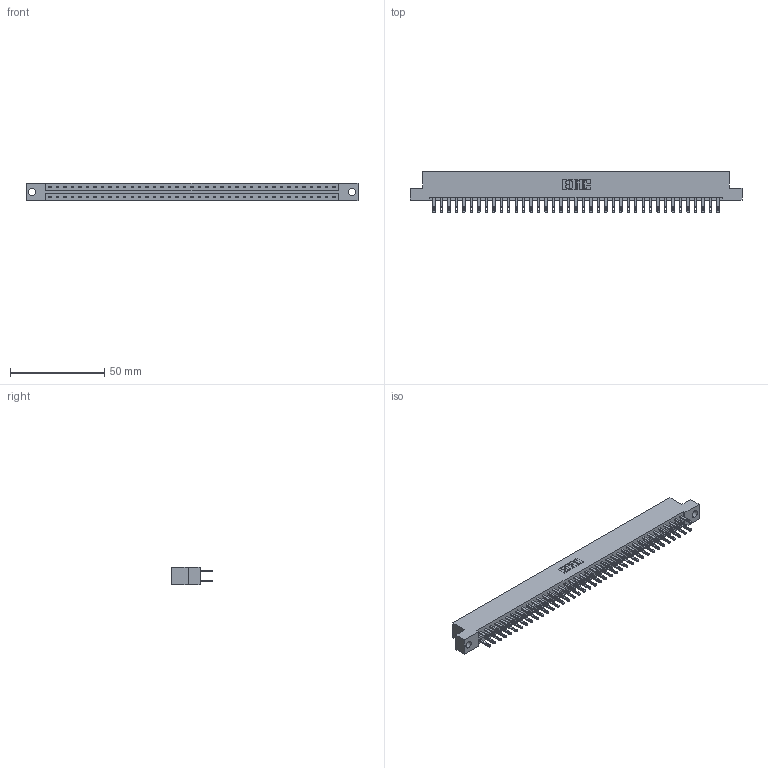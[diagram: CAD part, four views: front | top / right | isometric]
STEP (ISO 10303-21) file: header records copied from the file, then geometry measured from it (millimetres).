
FILE_DESCRIPTION (( 'STEP AP203' ), '1' );
FILE_NAME ('333-078-500-204.STEP', '2018-08-04T23:46:27', ( '' ), ( '' ), 'SwSTEP 2.0', 'SolidWorks 2016', '' );
FILE_SCHEMA (( 'CONFIG_CONTROL_DESIGN' ));
Length unit declared in the file: inch
Products named in the file (3): 333 Part_Flush - .156 Dia - TH; 345-292-001_345-293-100; 333-078-500-204
Assembly tree (79 placements, depth 2):
  333-078-500-204
    333 Part_Flush - .156 Dia - TH
    345-292-001_345-293-100  x78
Bounding box: 176.07 x 21.85 x 9.4 mm (x, y, z)
Volume: 18098.5 mm3; surface area: 22022.4 mm2
Topology: 79 solids, 79 shells, 3858 faces, 11777 edges, 7850 vertices
Faces by surface type: plane 2410, cylinder 1448
Entity records: 25411 total; most frequent: CARTESIAN_POINT 4214, ORIENTED_EDGE 4150, DIRECTION 3607, EDGE_CURVE 2075, LINE 1943, VECTOR 1943, VERTEX_POINT 1382, AXIS2_PLACEMENT_3D 832
